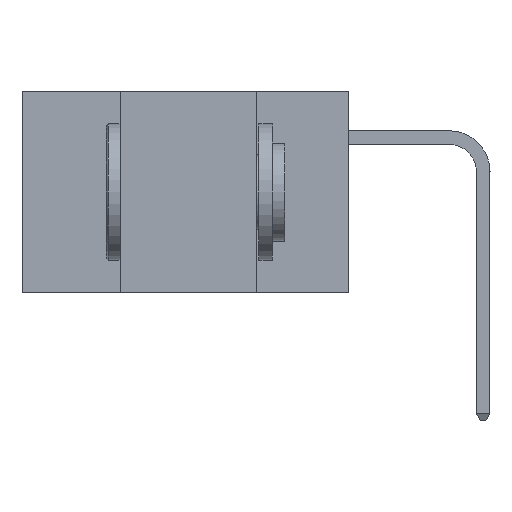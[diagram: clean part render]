
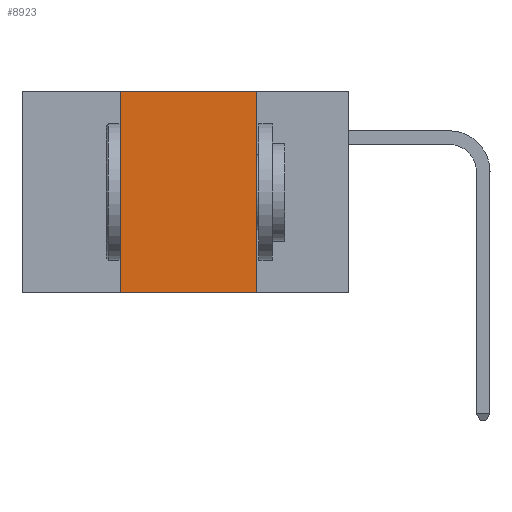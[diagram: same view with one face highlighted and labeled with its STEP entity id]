
A CAD part, left-side view. The second image highlights one B-rep face of the part: STEP entity #8923.
In plain terms, the highlighted planar face has unit normal (-1, 0, 0).
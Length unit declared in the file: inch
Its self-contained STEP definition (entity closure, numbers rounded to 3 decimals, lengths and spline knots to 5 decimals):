
#2213 = CARTESIAN_POINT ( 'NONE',  ( 0., 0.42, 0. ) ) ;
#3809 = AXIS2_PLACEMENT_3D ( 'NONE', #14712, #27846, #30290 ) ;
#5951 = CARTESIAN_POINT ( 'NONE',  ( 0., 0.42, 0. ) ) ;
#6341 = CARTESIAN_POINT ( 'NONE',  ( 0., 0.17, 0. ) ) ;
#6539 = LINE ( 'NONE', #6341, #33003 ) ;
#8923 = ADVANCED_FACE ( 'NONE', ( #21251 ), #21841, .F. ) ;
#9453 = DIRECTION ( 'NONE',  ( 0., 0., 1. ) ) ;
#9773 = DIRECTION ( 'NONE',  ( 0., -1., 0. ) ) ;
#10703 = CARTESIAN_POINT ( 'NONE',  ( 0., 0.17, 0. ) ) ;
#11783 = VECTOR ( 'NONE', #9773, 39.37008 ) ;
#12887 = CARTESIAN_POINT ( 'NONE',  ( 0., 0.6, -0.37 ) ) ;
#13726 = DIRECTION ( 'NONE',  ( 0., 0., -1. ) ) ;
#14633 = ORIENTED_EDGE ( 'NONE', *, *, #23015, .F. ) ;
#14712 = CARTESIAN_POINT ( 'NONE',  ( 0., 0.6, 0. ) ) ;
#16544 = EDGE_CURVE ( 'NONE', #25013, #19346, #37877, .T. ) ;
#17664 = LINE ( 'NONE', #2213, #36792 ) ;
#19346 = VERTEX_POINT ( 'NONE', #19633 ) ;
#19633 = CARTESIAN_POINT ( 'NONE',  ( 0., 0.17, -0.37 ) ) ;
#20331 = EDGE_LOOP ( 'NONE', ( #40175, #36022, #14633, #32555 ) ) ;
#20577 = VERTEX_POINT ( 'NONE', #10703 ) ;
#20633 = CARTESIAN_POINT ( 'NONE',  ( 0., 0.6, 0. ) ) ;
#21251 = FACE_OUTER_BOUND ( 'NONE', #20331, .T. ) ;
#21521 = EDGE_CURVE ( 'NONE', #42050, #20577, #30971, .T. ) ;
#21841 = PLANE ( 'NONE',  #3809 ) ;
#23015 = EDGE_CURVE ( 'NONE', #25013, #42050, #17664, .T. ) ;
#25013 = VERTEX_POINT ( 'NONE', #38367 ) ;
#26780 = DIRECTION ( 'NONE',  ( 0., -1., 0. ) ) ;
#27846 = DIRECTION ( 'NONE',  ( 1., 0., 0. ) ) ;
#30290 = DIRECTION ( 'NONE',  ( 0., 0., -1. ) ) ;
#30971 = LINE ( 'NONE', #20633, #11783 ) ;
#32555 = ORIENTED_EDGE ( 'NONE', *, *, #16544, .T. ) ;
#33003 = VECTOR ( 'NONE', #13726, 39.37008 ) ;
#36022 = ORIENTED_EDGE ( 'NONE', *, *, #21521, .F. ) ;
#36792 = VECTOR ( 'NONE', #9453, 39.37008 ) ;
#37877 = LINE ( 'NONE', #12887, #45199 ) ;
#38367 = CARTESIAN_POINT ( 'NONE',  ( 0., 0.42, -0.37 ) ) ;
#40175 = ORIENTED_EDGE ( 'NONE', *, *, #46345, .F. ) ;
#42050 = VERTEX_POINT ( 'NONE', #5951 ) ;
#45199 = VECTOR ( 'NONE', #26780, 39.37008 ) ;
#46345 = EDGE_CURVE ( 'NONE', #20577, #19346, #6539, .T. ) ;
